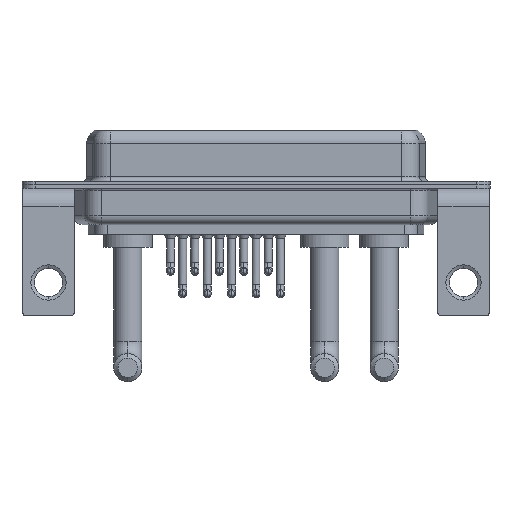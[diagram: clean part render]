
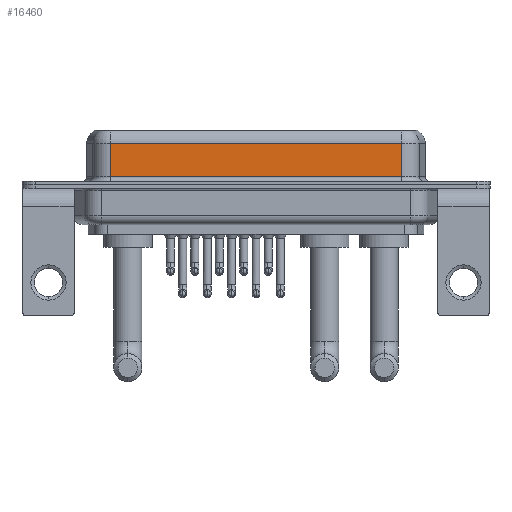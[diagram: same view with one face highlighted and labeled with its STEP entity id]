
A CAD part, front view. The second image highlights one B-rep face of the part: STEP entity #16460.
In plain terms, the highlighted planar face has unit normal (0, -1, 0).
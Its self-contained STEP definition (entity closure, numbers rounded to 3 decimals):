
#305 = CARTESIAN_POINT ( 'NONE',  ( 7.013, -3.95, 4.65 ) ) ;
#388 = DIRECTION ( 'NONE',  ( 0., 0., -1. ) ) ;
#676 = CARTESIAN_POINT ( 'NONE',  ( 7.013, -3.95, 6.4 ) ) ;
#1352 = CARTESIAN_POINT ( 'NONE',  ( 40.037, -3.95, 0.9 ) ) ;
#2219 = DIRECTION ( 'NONE',  ( 0., 0., -1. ) ) ;
#3250 = VECTOR ( 'NONE', #2219, 1000. ) ;
#3691 = ORIENTED_EDGE ( 'NONE', *, *, #14045, .T. ) ;
#4297 = AXIS2_PLACEMENT_3D ( 'NONE', #14397, #12369, #18509 ) ;
#4876 = VECTOR ( 'NONE', #388, 1000. ) ;
#5483 = CARTESIAN_POINT ( 'NONE',  ( 40.037, -3.95, 0.9 ) ) ;
#6275 = CARTESIAN_POINT ( 'NONE',  ( 40.037, -3.95, 4.65 ) ) ;
#7208 = ORIENTED_EDGE ( 'NONE', *, *, #13039, .F. ) ;
#7222 = EDGE_CURVE ( 'NONE', #19559, #10995, #9898, .T. ) ;
#7539 = VECTOR ( 'NONE', #14550, 1000. ) ;
#7605 = DIRECTION ( 'NONE',  ( -1., 0., 0. ) ) ;
#7700 = CARTESIAN_POINT ( 'NONE',  ( 40.037, -3.95, 4.65 ) ) ;
#8097 = VECTOR ( 'NONE', #7605, 1000. ) ;
#8133 = CARTESIAN_POINT ( 'NONE',  ( 40.037, -3.95, 6.4 ) ) ;
#8251 = PLANE ( 'NONE',  #4297 ) ;
#9898 = LINE ( 'NONE', #5483, #7539 ) ;
#10576 = LINE ( 'NONE', #8133, #3250 ) ;
#10995 = VERTEX_POINT ( 'NONE', #1352 ) ;
#12369 = DIRECTION ( 'NONE',  ( 0., 1., 0. ) ) ;
#12553 = ORIENTED_EDGE ( 'NONE', *, *, #7222, .T. ) ;
#12581 = VERTEX_POINT ( 'NONE', #6275 ) ;
#12626 = CARTESIAN_POINT ( 'NONE',  ( 7.013, -3.95, 0.9 ) ) ;
#13039 = EDGE_CURVE ( 'NONE', #12581, #10995, #10576, .T. ) ;
#14045 = EDGE_CURVE ( 'NONE', #12581, #18221, #16849, .T. ) ;
#14137 = LINE ( 'NONE', #676, #4876 ) ;
#14161 = EDGE_CURVE ( 'NONE', #18221, #19559, #14137, .T. ) ;
#14190 = FACE_OUTER_BOUND ( 'NONE', #14383, .T. ) ;
#14383 = EDGE_LOOP ( 'NONE', ( #7208, #3691, #19593, #12553 ) ) ;
#14397 = CARTESIAN_POINT ( 'NONE',  ( 40.037, -3.95, 6.4 ) ) ;
#14550 = DIRECTION ( 'NONE',  ( 1., 0., 0. ) ) ;
#16460 = ADVANCED_FACE ( 'NONE', ( #14190 ), #8251, .F. ) ;
#16849 = LINE ( 'NONE', #7700, #8097 ) ;
#18221 = VERTEX_POINT ( 'NONE', #305 ) ;
#18509 = DIRECTION ( 'NONE',  ( 0., 0., 1. ) ) ;
#19559 = VERTEX_POINT ( 'NONE', #12626 ) ;
#19593 = ORIENTED_EDGE ( 'NONE', *, *, #14161, .T. ) ;
